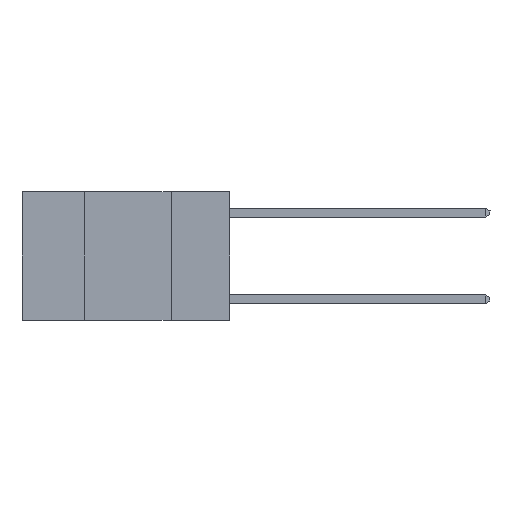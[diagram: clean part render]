
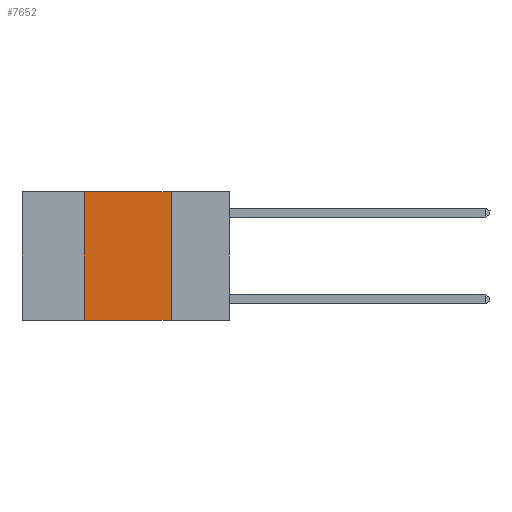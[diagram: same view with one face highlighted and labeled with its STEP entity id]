
A CAD part, left-side view. The second image highlights one B-rep face of the part: STEP entity #7652.
In plain terms, the highlighted planar face has unit normal (-1, 0, 0).
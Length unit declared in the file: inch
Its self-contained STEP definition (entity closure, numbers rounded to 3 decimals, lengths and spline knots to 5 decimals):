
#263 = EDGE_LOOP ( 'NONE', ( #12415, #12399, #5245, #6697 ) ) ;
#784 = CARTESIAN_POINT ( 'NONE',  ( 0., 0.17, 0. ) ) ;
#1098 = VERTEX_POINT ( 'NONE', #5398 ) ;
#1760 = LINE ( 'NONE', #11151, #10740 ) ;
#2132 = DIRECTION ( 'NONE',  ( 1., 0., 0. ) ) ;
#2728 = VECTOR ( 'NONE', #6786, 39.37008 ) ;
#2844 = EDGE_CURVE ( 'NONE', #5404, #4185, #1760, .T. ) ;
#3218 = PLANE ( 'NONE',  #10752 ) ;
#3644 = LINE ( 'NONE', #12003, #2728 ) ;
#4185 = VERTEX_POINT ( 'NONE', #8995 ) ;
#4327 = CARTESIAN_POINT ( 'NONE',  ( 0., 0.42, 0. ) ) ;
#5196 = FACE_OUTER_BOUND ( 'NONE', #263, .T. ) ;
#5245 = ORIENTED_EDGE ( 'NONE', *, *, #5339, .F. ) ;
#5339 = EDGE_CURVE ( 'NONE', #10140, #5404, #3644, .T. ) ;
#5398 = CARTESIAN_POINT ( 'NONE',  ( 0., 0.17, -0.37 ) ) ;
#5404 = VERTEX_POINT ( 'NONE', #4327 ) ;
#6343 = DIRECTION ( 'NONE',  ( 0., 0., -1. ) ) ;
#6697 = ORIENTED_EDGE ( 'NONE', *, *, #11898, .T. ) ;
#6786 = DIRECTION ( 'NONE',  ( 0., 0., 1. ) ) ;
#7140 = EDGE_CURVE ( 'NONE', #4185, #1098, #11186, .T. ) ;
#7221 = DIRECTION ( 'NONE',  ( 0., -1., 0. ) ) ;
#7652 = ADVANCED_FACE ( 'NONE', ( #5196 ), #3218, .F. ) ;
#8602 = VECTOR ( 'NONE', #7221, 39.37008 ) ;
#8735 = VECTOR ( 'NONE', #11068, 39.37008 ) ;
#8995 = CARTESIAN_POINT ( 'NONE',  ( 0., 0.17, 0. ) ) ;
#9349 = LINE ( 'NONE', #13432, #8602 ) ;
#9372 = CARTESIAN_POINT ( 'NONE',  ( 0., 0.6, 0. ) ) ;
#10140 = VERTEX_POINT ( 'NONE', #12865 ) ;
#10740 = VECTOR ( 'NONE', #12422, 39.37008 ) ;
#10752 = AXIS2_PLACEMENT_3D ( 'NONE', #9372, #2132, #6343 ) ;
#11068 = DIRECTION ( 'NONE',  ( 0., 0., -1. ) ) ;
#11151 = CARTESIAN_POINT ( 'NONE',  ( 0., 0.6, 0. ) ) ;
#11186 = LINE ( 'NONE', #784, #8735 ) ;
#11898 = EDGE_CURVE ( 'NONE', #10140, #1098, #9349, .T. ) ;
#12003 = CARTESIAN_POINT ( 'NONE',  ( 0., 0.42, 0. ) ) ;
#12399 = ORIENTED_EDGE ( 'NONE', *, *, #2844, .F. ) ;
#12415 = ORIENTED_EDGE ( 'NONE', *, *, #7140, .F. ) ;
#12422 = DIRECTION ( 'NONE',  ( 0., -1., 0. ) ) ;
#12865 = CARTESIAN_POINT ( 'NONE',  ( 0., 0.42, -0.37 ) ) ;
#13432 = CARTESIAN_POINT ( 'NONE',  ( 0., 0.6, -0.37 ) ) ;
